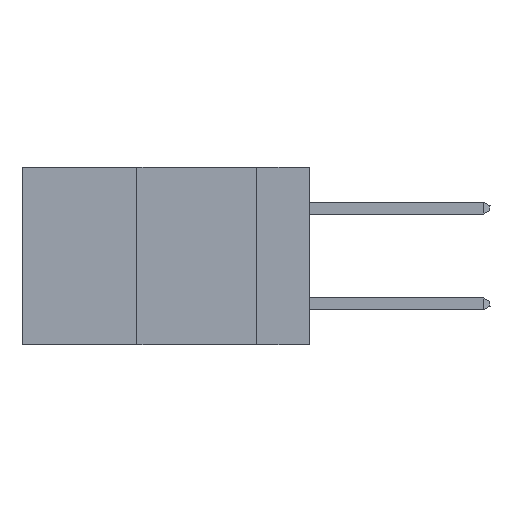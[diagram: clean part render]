
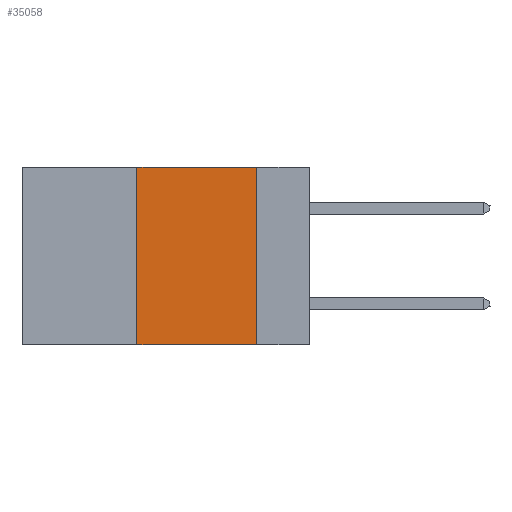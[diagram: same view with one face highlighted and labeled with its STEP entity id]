
A CAD part, left-side view. The second image highlights one B-rep face of the part: STEP entity #35058.
In plain terms, the highlighted planar face has unit normal (-1, 0, 0).
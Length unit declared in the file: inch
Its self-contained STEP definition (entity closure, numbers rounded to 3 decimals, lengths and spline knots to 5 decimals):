
#259 = DIRECTION ( 'NONE',  ( 0., 0., 1. ) ) ;
#415 = VECTOR ( 'NONE', #25240, 39.37008 ) ;
#668 = EDGE_CURVE ( 'NONE', #1733, #9918, #19786, .T. ) ;
#717 = PLANE ( 'NONE',  #26728 ) ;
#1733 = VERTEX_POINT ( 'NONE', #30709 ) ;
#2614 = CARTESIAN_POINT ( 'NONE',  ( 0., 0.11, 0. ) ) ;
#2865 = EDGE_CURVE ( 'NONE', #9918, #19971, #36673, .T. ) ;
#3327 = FACE_OUTER_BOUND ( 'NONE', #41576, .T. ) ;
#3642 = ORIENTED_EDGE ( 'NONE', *, *, #2865, .F. ) ;
#4393 = ORIENTED_EDGE ( 'NONE', *, *, #15551, .F. ) ;
#4400 = CARTESIAN_POINT ( 'NONE',  ( 0., 0.6, 0. ) ) ;
#5472 = VERTEX_POINT ( 'NONE', #16122 ) ;
#5694 = VECTOR ( 'NONE', #38753, 39.37008 ) ;
#7096 = DIRECTION ( 'NONE',  ( 0., 0., -1. ) ) ;
#9918 = VERTEX_POINT ( 'NONE', #16677 ) ;
#11257 = CARTESIAN_POINT ( 'NONE',  ( 0., 0.6, 0. ) ) ;
#15551 = EDGE_CURVE ( 'NONE', #19971, #5472, #28100, .T. ) ;
#16122 = CARTESIAN_POINT ( 'NONE',  ( 0., 0.11, -0.37 ) ) ;
#16677 = CARTESIAN_POINT ( 'NONE',  ( 0., 0.36, 0. ) ) ;
#16998 = DIRECTION ( 'NONE',  ( 1., 0., 0. ) ) ;
#18709 = EDGE_CURVE ( 'NONE', #1733, #5472, #27808, .T. ) ;
#19579 = VECTOR ( 'NONE', #27381, 39.37008 ) ;
#19786 = LINE ( 'NONE', #31750, #40894 ) ;
#19971 = VERTEX_POINT ( 'NONE', #29377 ) ;
#23084 = ORIENTED_EDGE ( 'NONE', *, *, #668, .F. ) ;
#25240 = DIRECTION ( 'NONE',  ( 0., 0., -1. ) ) ;
#26728 = AXIS2_PLACEMENT_3D ( 'NONE', #4400, #16998, #7096 ) ;
#27381 = DIRECTION ( 'NONE',  ( 0., -1., 0. ) ) ;
#27808 = LINE ( 'NONE', #41547, #5694 ) ;
#28100 = LINE ( 'NONE', #2614, #415 ) ;
#29377 = CARTESIAN_POINT ( 'NONE',  ( 0., 0.11, 0. ) ) ;
#29996 = ORIENTED_EDGE ( 'NONE', *, *, #18709, .T. ) ;
#30709 = CARTESIAN_POINT ( 'NONE',  ( 0., 0.36, -0.37 ) ) ;
#31750 = CARTESIAN_POINT ( 'NONE',  ( 0., 0.36, 0. ) ) ;
#35058 = ADVANCED_FACE ( 'NONE', ( #3327 ), #717, .F. ) ;
#36673 = LINE ( 'NONE', #11257, #19579 ) ;
#38753 = DIRECTION ( 'NONE',  ( 0., -1., 0. ) ) ;
#40894 = VECTOR ( 'NONE', #259, 39.37008 ) ;
#41547 = CARTESIAN_POINT ( 'NONE',  ( 0., 0.6, -0.37 ) ) ;
#41576 = EDGE_LOOP ( 'NONE', ( #4393, #3642, #23084, #29996 ) ) ;
